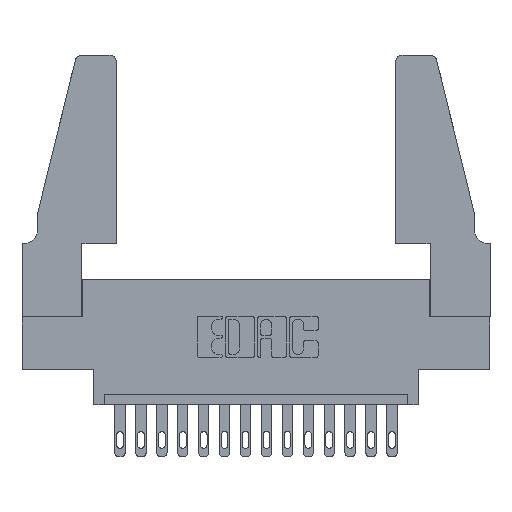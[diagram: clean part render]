
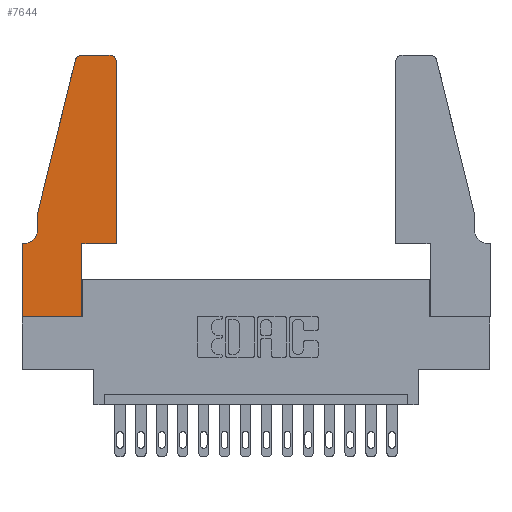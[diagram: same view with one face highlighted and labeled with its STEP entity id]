
A CAD part, top view. The second image highlights one B-rep face of the part: STEP entity #7644.
In plain terms, the highlighted planar face has unit normal (0, 0, 1).
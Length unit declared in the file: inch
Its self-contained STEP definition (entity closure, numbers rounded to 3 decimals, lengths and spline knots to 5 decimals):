
#59 = VECTOR ( 'NONE', #12045, 39.37008 ) ;
#106 = EDGE_CURVE ( 'NONE', #9916, #6292, #10896, .T. ) ;
#613 = ORIENTED_EDGE ( 'NONE', *, *, #14292, .T. ) ;
#963 = CIRCLE ( 'NONE', #12183, 0.07 ) ;
#994 = CARTESIAN_POINT ( 'NONE',  ( 0.0755, 0.5, 0.37 ) ) ;
#1208 = DIRECTION ( 'NONE',  ( -1., 0., 0. ) ) ;
#1281 = VECTOR ( 'NONE', #2534, 39.37008 ) ;
#1324 = VERTEX_POINT ( 'NONE', #5814 ) ;
#1603 = DIRECTION ( 'NONE',  ( -0.239, -0.971, 0. ) ) ;
#1661 = DIRECTION ( 'NONE',  ( 1., 0., 0. ) ) ;
#1927 = CARTESIAN_POINT ( 'NONE',  ( 0.4505, 1.22, 0.37 ) ) ;
#2264 = ORIENTED_EDGE ( 'NONE', *, *, #5366, .T. ) ;
#2314 = EDGE_CURVE ( 'NONE', #9119, #15692, #12403, .T. ) ;
#2483 = CARTESIAN_POINT ( 'NONE',  ( 0.0755, 0.42, 0.37 ) ) ;
#2534 = DIRECTION ( 'NONE',  ( 1., 0., 0. ) ) ;
#2987 = VECTOR ( 'NONE', #5673, 39.37008 ) ;
#3040 = CIRCLE ( 'NONE', #9520, 0.03 ) ;
#3117 = EDGE_CURVE ( 'NONE', #8004, #12617, #4789, .T. ) ;
#3178 = EDGE_CURVE ( 'NONE', #12522, #12606, #963, .T. ) ;
#3206 = ORIENTED_EDGE ( 'NONE', *, *, #2314, .T. ) ;
#3405 = DIRECTION ( 'NONE',  ( 0., 0., 1. ) ) ;
#3523 = DIRECTION ( 'NONE',  ( 1., 0., 0. ) ) ;
#3869 = CARTESIAN_POINT ( 'NONE',  ( 0., 0., 0.37 ) ) ;
#3892 = CARTESIAN_POINT ( 'NONE',  ( 0.0755, 0.35, 0.37 ) ) ;
#4184 = CARTESIAN_POINT ( 'NONE',  ( 0.4205, 1.22, 0.37 ) ) ;
#4391 = CARTESIAN_POINT ( 'NONE',  ( 0., 0., 0.37 ) ) ;
#4541 = VECTOR ( 'NONE', #3523, 39.37008 ) ;
#4710 = CARTESIAN_POINT ( 'NONE',  ( 0.2605, 1.25, 0.37 ) ) ;
#4726 = CARTESIAN_POINT ( 'NONE',  ( 0.4505, 0.35, 0.37 ) ) ;
#4789 = LINE ( 'NONE', #4710, #6179 ) ;
#4814 = CARTESIAN_POINT ( 'NONE',  ( 0.2865, 0.35, 0.37 ) ) ;
#4886 = VERTEX_POINT ( 'NONE', #10917 ) ;
#5000 = CARTESIAN_POINT ( 'NONE',  ( 0.0755, 0.5, 0.37 ) ) ;
#5021 = EDGE_CURVE ( 'NONE', #9087, #9916, #7558, .T. ) ;
#5366 = EDGE_CURVE ( 'NONE', #1324, #4886, #10311, .T. ) ;
#5673 = DIRECTION ( 'NONE',  ( 0., -1., 0. ) ) ;
#5710 = AXIS2_PLACEMENT_3D ( 'NONE', #13286, #15645, #1661 ) ;
#5814 = CARTESIAN_POINT ( 'NONE',  ( 0., 0., 0.37 ) ) ;
#5910 = CARTESIAN_POINT ( 'NONE',  ( 0.284, 1.22, 0.37 ) ) ;
#6179 = VECTOR ( 'NONE', #9791, 39.37008 ) ;
#6292 = VERTEX_POINT ( 'NONE', #1927 ) ;
#6322 = DIRECTION ( 'NONE',  ( -1., 0., 0. ) ) ;
#6629 = ORIENTED_EDGE ( 'NONE', *, *, #9023, .T. ) ;
#6651 = CIRCLE ( 'NONE', #7029, 0.03 ) ;
#6914 = CARTESIAN_POINT ( 'NONE',  ( 0.0755, 0.5, 0.37 ) ) ;
#6992 = CARTESIAN_POINT ( 'NONE',  ( 0.2865, 0.35, 0.37 ) ) ;
#7024 = CARTESIAN_POINT ( 'NONE',  ( 0.284, 1.25, 0.37 ) ) ;
#7029 = AXIS2_PLACEMENT_3D ( 'NONE', #4184, #12003, #8163 ) ;
#7239 = LINE ( 'NONE', #4391, #2987 ) ;
#7311 = CARTESIAN_POINT ( 'NONE',  ( 0.25487, 1.22718, 0.37 ) ) ;
#7340 = CARTESIAN_POINT ( 'NONE',  ( 0.4205, 1.25, 0.37 ) ) ;
#7558 = LINE ( 'NONE', #4726, #4541 ) ;
#7644 = ADVANCED_FACE ( 'NONE', ( #10038 ), #10469, .T. ) ;
#8004 = VERTEX_POINT ( 'NONE', #7340 ) ;
#8027 = LINE ( 'NONE', #994, #8822 ) ;
#8163 = DIRECTION ( 'NONE',  ( 1., 0., 0. ) ) ;
#8235 = EDGE_CURVE ( 'NONE', #6292, #8004, #6651, .T. ) ;
#8676 = DIRECTION ( 'NONE',  ( 1., 0., 0. ) ) ;
#8822 = VECTOR ( 'NONE', #13662, 39.37008 ) ;
#9023 = EDGE_CURVE ( 'NONE', #14010, #1324, #7239, .T. ) ;
#9087 = VERTEX_POINT ( 'NONE', #6992 ) ;
#9119 = VERTEX_POINT ( 'NONE', #7311 ) ;
#9271 = CARTESIAN_POINT ( 'NONE',  ( 0., 0.35, 0.37 ) ) ;
#9520 = AXIS2_PLACEMENT_3D ( 'NONE', #5910, #3405, #8676 ) ;
#9791 = DIRECTION ( 'NONE',  ( -1., 0., 0. ) ) ;
#9916 = VERTEX_POINT ( 'NONE', #13547 ) ;
#10038 = FACE_OUTER_BOUND ( 'NONE', #11310, .T. ) ;
#10311 = LINE ( 'NONE', #3869, #1281 ) ;
#10447 = ORIENTED_EDGE ( 'NONE', *, *, #16434, .T. ) ;
#10469 = PLANE ( 'NONE',  #5710 ) ;
#10857 = CARTESIAN_POINT ( 'NONE',  ( 0.0055, 0.35, 0.37 ) ) ;
#10896 = LINE ( 'NONE', #13267, #59 ) ;
#10917 = CARTESIAN_POINT ( 'NONE',  ( 0.2865, 0., 0.37 ) ) ;
#11047 = ORIENTED_EDGE ( 'NONE', *, *, #3178, .T. ) ;
#11121 = LINE ( 'NONE', #3892, #13884 ) ;
#11229 = DIRECTION ( 'NONE',  ( 0., 1., 0. ) ) ;
#11310 = EDGE_LOOP ( 'NONE', ( #14633, #15263, #3206, #10447, #11047, #14056, #6629, #2264, #613, #15556, #12486, #13648 ) ) ;
#11606 = CARTESIAN_POINT ( 'NONE',  ( 0.0055, 0.42, 0.37 ) ) ;
#12003 = DIRECTION ( 'NONE',  ( 0., 0., 1. ) ) ;
#12045 = DIRECTION ( 'NONE',  ( 0., 1., 0. ) ) ;
#12183 = AXIS2_PLACEMENT_3D ( 'NONE', #11606, #16498, #6322 ) ;
#12403 = LINE ( 'NONE', #6914, #13765 ) ;
#12486 = ORIENTED_EDGE ( 'NONE', *, *, #106, .T. ) ;
#12522 = VERTEX_POINT ( 'NONE', #2483 ) ;
#12606 = VERTEX_POINT ( 'NONE', #10857 ) ;
#12617 = VERTEX_POINT ( 'NONE', #7024 ) ;
#12865 = VECTOR ( 'NONE', #11229, 39.37008 ) ;
#13267 = CARTESIAN_POINT ( 'NONE',  ( 0.4505, 0.35, 0.37 ) ) ;
#13286 = CARTESIAN_POINT ( 'NONE',  ( 0., 0.35, 0.37 ) ) ;
#13547 = CARTESIAN_POINT ( 'NONE',  ( 0.4505, 0.35, 0.37 ) ) ;
#13648 = ORIENTED_EDGE ( 'NONE', *, *, #8235, .T. ) ;
#13662 = DIRECTION ( 'NONE',  ( 0., -1., 0. ) ) ;
#13765 = VECTOR ( 'NONE', #1603, 39.37008 ) ;
#13850 = EDGE_CURVE ( 'NONE', #12606, #14010, #11121, .T. ) ;
#13884 = VECTOR ( 'NONE', #1208, 39.37008 ) ;
#14010 = VERTEX_POINT ( 'NONE', #9271 ) ;
#14056 = ORIENTED_EDGE ( 'NONE', *, *, #13850, .T. ) ;
#14292 = EDGE_CURVE ( 'NONE', #4886, #9087, #14435, .T. ) ;
#14435 = LINE ( 'NONE', #4814, #12865 ) ;
#14633 = ORIENTED_EDGE ( 'NONE', *, *, #3117, .T. ) ;
#15263 = ORIENTED_EDGE ( 'NONE', *, *, #15412, .T. ) ;
#15412 = EDGE_CURVE ( 'NONE', #12617, #9119, #3040, .T. ) ;
#15556 = ORIENTED_EDGE ( 'NONE', *, *, #5021, .T. ) ;
#15645 = DIRECTION ( 'NONE',  ( 0., 0., 1. ) ) ;
#15692 = VERTEX_POINT ( 'NONE', #5000 ) ;
#16434 = EDGE_CURVE ( 'NONE', #15692, #12522, #8027, .T. ) ;
#16498 = DIRECTION ( 'NONE',  ( 0., 0., -1. ) ) ;
